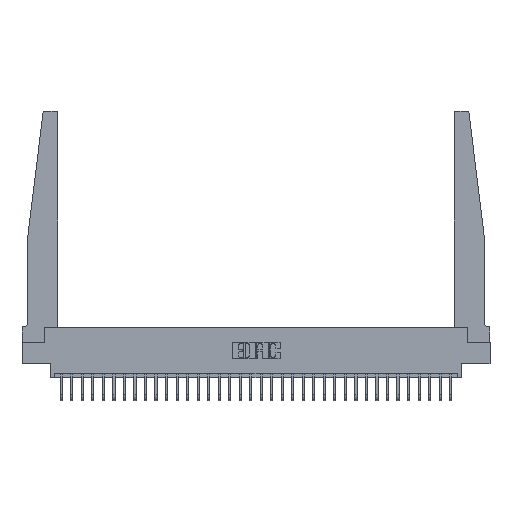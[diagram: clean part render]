
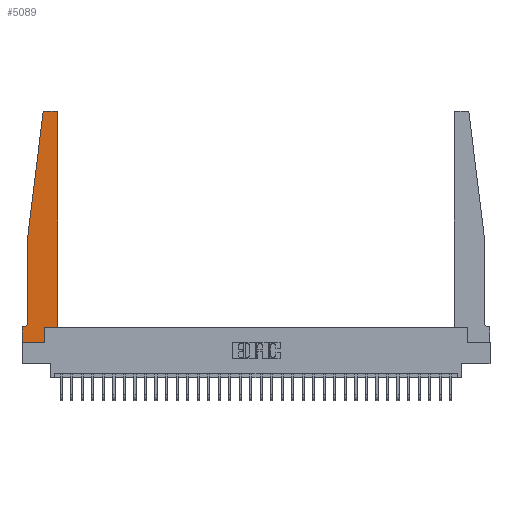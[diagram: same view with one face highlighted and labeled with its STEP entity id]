
A CAD part, top view. The second image highlights one B-rep face of the part: STEP entity #5089.
In plain terms, the highlighted planar face has unit normal (0, 0, 1).
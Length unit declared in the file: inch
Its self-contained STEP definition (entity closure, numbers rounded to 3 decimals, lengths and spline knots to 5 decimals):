
#339 = EDGE_CURVE ( 'NONE', #12382, #13331, #5246, .T. ) ;
#435 = FACE_OUTER_BOUND ( 'NONE', #11037, .T. ) ;
#787 = VERTEX_POINT ( 'NONE', #13876 ) ;
#1218 = VECTOR ( 'NONE', #23443, 39.37008 ) ;
#1477 = CARTESIAN_POINT ( 'NONE',  ( 0.395, 2.72, 0.37 ) ) ;
#1482 = DIRECTION ( 'NONE',  ( -1., 0., 0. ) ) ;
#1632 = CARTESIAN_POINT ( 'NONE',  ( 0., 0., 0.37 ) ) ;
#1955 = LINE ( 'NONE', #21192, #1218 ) ;
#2111 = ORIENTED_EDGE ( 'NONE', *, *, #27440, .T. ) ;
#2190 = LINE ( 'NONE', #15433, #6166 ) ;
#2281 = EDGE_CURVE ( 'NONE', #15164, #2390, #3346, .T. ) ;
#2390 = VERTEX_POINT ( 'NONE', #8690 ) ;
#2768 = CARTESIAN_POINT ( 'NONE',  ( 0.425, 2.72, 0.37 ) ) ;
#2798 = VERTEX_POINT ( 'NONE', #14584 ) ;
#3346 = LINE ( 'NONE', #19390, #26452 ) ;
#3579 = CARTESIAN_POINT ( 'NONE',  ( 0.2605, 0.18, 0.37 ) ) ;
#3644 = EDGE_CURVE ( 'NONE', #13331, #2798, #2190, .T. ) ;
#3822 = DIRECTION ( 'NONE',  ( 1., 0., 0. ) ) ;
#3839 = VECTOR ( 'NONE', #19632, 39.37008 ) ;
#3952 = DIRECTION ( 'NONE',  ( 0., 0., -1. ) ) ;
#4383 = ORIENTED_EDGE ( 'NONE', *, *, #16324, .T. ) ;
#4418 = DIRECTION ( 'NONE',  ( 0., 0., 1. ) ) ;
#4442 = ORIENTED_EDGE ( 'NONE', *, *, #9662, .T. ) ;
#4930 = CARTESIAN_POINT ( 'NONE',  ( 0.065, 1.25, 0.37 ) ) ;
#5016 = VERTEX_POINT ( 'NONE', #24161 ) ;
#5089 = ADVANCED_FACE ( 'NONE', ( #435 ), #15569, .T. ) ;
#5246 = LINE ( 'NONE', #3579, #22359 ) ;
#5272 = AXIS2_PLACEMENT_3D ( 'NONE', #22437, #9103, #24684 ) ;
#5592 = ORIENTED_EDGE ( 'NONE', *, *, #10603, .T. ) ;
#6166 = VECTOR ( 'NONE', #11150, 39.37008 ) ;
#7247 = CARTESIAN_POINT ( 'NONE',  ( 0.395, 2.75, 0.37 ) ) ;
#7549 = ORIENTED_EDGE ( 'NONE', *, *, #24615, .T. ) ;
#8267 = CARTESIAN_POINT ( 'NONE',  ( 0.065, 1.25, 0.37 ) ) ;
#8557 = LINE ( 'NONE', #25179, #19693 ) ;
#8690 = CARTESIAN_POINT ( 'NONE',  ( 0., 0.1875, 0.37 ) ) ;
#9103 = DIRECTION ( 'NONE',  ( 0., 0., 1. ) ) ;
#9288 = CARTESIAN_POINT ( 'NONE',  ( 0.25, 2.75, 0.37 ) ) ;
#9388 = CARTESIAN_POINT ( 'NONE',  ( 0.2605, 0., 0.37 ) ) ;
#9662 = EDGE_CURVE ( 'NONE', #21662, #10698, #18892, .T. ) ;
#10601 = CIRCLE ( 'NONE', #15765, 0.05 ) ;
#10603 = EDGE_CURVE ( 'NONE', #5016, #787, #27200, .T. ) ;
#10657 = EDGE_CURVE ( 'NONE', #10698, #5016, #14660, .T. ) ;
#10698 = VERTEX_POINT ( 'NONE', #7247 ) ;
#11037 = EDGE_LOOP ( 'NONE', ( #26169, #5592, #16190, #2111, #7549, #25469, #4383, #26163, #25231, #12651, #22467, #4442 ) ) ;
#11150 = DIRECTION ( 'NONE',  ( 1., 0., 0. ) ) ;
#11253 = LINE ( 'NONE', #4930, #21707 ) ;
#12382 = VERTEX_POINT ( 'NONE', #9388 ) ;
#12464 = CARTESIAN_POINT ( 'NONE',  ( 0.065, 0.2375, 0.37 ) ) ;
#12651 = ORIENTED_EDGE ( 'NONE', *, *, #3644, .T. ) ;
#12774 = LINE ( 'NONE', #13420, #18703 ) ;
#13331 = VERTEX_POINT ( 'NONE', #28019 ) ;
#13420 = CARTESIAN_POINT ( 'NONE',  ( 0., 0., 0.37 ) ) ;
#13876 = CARTESIAN_POINT ( 'NONE',  ( 0.24675, 2.72367, 0.37 ) ) ;
#14417 = AXIS2_PLACEMENT_3D ( 'NONE', #1477, #17260, #3822 ) ;
#14584 = CARTESIAN_POINT ( 'NONE',  ( 0.425, 0.18, 0.37 ) ) ;
#14660 = LINE ( 'NONE', #9288, #25820 ) ;
#15164 = VERTEX_POINT ( 'NONE', #19378 ) ;
#15433 = CARTESIAN_POINT ( 'NONE',  ( 0.425, 0.18, 0.37 ) ) ;
#15569 = PLANE ( 'NONE',  #17162 ) ;
#15765 = AXIS2_PLACEMENT_3D ( 'NONE', #17368, #3952, #19611 ) ;
#15772 = LINE ( 'NONE', #1632, #3839 ) ;
#15847 = VERTEX_POINT ( 'NONE', #18084 ) ;
#16190 = ORIENTED_EDGE ( 'NONE', *, *, #25506, .T. ) ;
#16324 = EDGE_CURVE ( 'NONE', #2390, #15847, #15772, .T. ) ;
#17162 = AXIS2_PLACEMENT_3D ( 'NONE', #24457, #4418, #20051 ) ;
#17260 = DIRECTION ( 'NONE',  ( 0., 0., 1. ) ) ;
#17368 = CARTESIAN_POINT ( 'NONE',  ( 0.015, 0.2375, 0.37 ) ) ;
#18084 = CARTESIAN_POINT ( 'NONE',  ( 0., 0., 0.37 ) ) ;
#18703 = VECTOR ( 'NONE', #28998, 39.37008 ) ;
#18892 = CIRCLE ( 'NONE', #14417, 0.03 ) ;
#19264 = DIRECTION ( 'NONE',  ( 0., 1., 0. ) ) ;
#19378 = CARTESIAN_POINT ( 'NONE',  ( 0.015, 0.1875, 0.37 ) ) ;
#19390 = CARTESIAN_POINT ( 'NONE',  ( 0.065, 0.1875, 0.37 ) ) ;
#19611 = DIRECTION ( 'NONE',  ( -1., 0., 0. ) ) ;
#19632 = DIRECTION ( 'NONE',  ( 0., -1., 0. ) ) ;
#19693 = VECTOR ( 'NONE', #27398, 39.37008 ) ;
#20051 = DIRECTION ( 'NONE',  ( 1., 0., 0. ) ) ;
#20358 = VERTEX_POINT ( 'NONE', #12464 ) ;
#21192 = CARTESIAN_POINT ( 'NONE',  ( 0.065, 1.25, 0.37 ) ) ;
#21662 = VERTEX_POINT ( 'NONE', #2768 ) ;
#21707 = VECTOR ( 'NONE', #25409, 39.37008 ) ;
#22359 = VECTOR ( 'NONE', #19264, 39.37008 ) ;
#22437 = CARTESIAN_POINT ( 'NONE',  ( 0.27653, 2.72, 0.37 ) ) ;
#22467 = ORIENTED_EDGE ( 'NONE', *, *, #24278, .T. ) ;
#23201 = EDGE_CURVE ( 'NONE', #15847, #12382, #12774, .T. ) ;
#23443 = DIRECTION ( 'NONE',  ( 0., -1., 0. ) ) ;
#23915 = VERTEX_POINT ( 'NONE', #8267 ) ;
#24161 = CARTESIAN_POINT ( 'NONE',  ( 0.27653, 2.75, 0.37 ) ) ;
#24278 = EDGE_CURVE ( 'NONE', #2798, #21662, #8557, .T. ) ;
#24457 = CARTESIAN_POINT ( 'NONE',  ( 0., 0.1875, 0.37 ) ) ;
#24615 = EDGE_CURVE ( 'NONE', #20358, #15164, #10601, .T. ) ;
#24684 = DIRECTION ( 'NONE',  ( 1., 0., 0. ) ) ;
#24869 = DIRECTION ( 'NONE',  ( -1., 0., 0. ) ) ;
#25179 = CARTESIAN_POINT ( 'NONE',  ( 0.425, 0.18, 0.37 ) ) ;
#25231 = ORIENTED_EDGE ( 'NONE', *, *, #339, .T. ) ;
#25409 = DIRECTION ( 'NONE',  ( -0.122, -0.992, 0. ) ) ;
#25469 = ORIENTED_EDGE ( 'NONE', *, *, #2281, .T. ) ;
#25506 = EDGE_CURVE ( 'NONE', #787, #23915, #11253, .T. ) ;
#25820 = VECTOR ( 'NONE', #24869, 39.37008 ) ;
#26163 = ORIENTED_EDGE ( 'NONE', *, *, #23201, .T. ) ;
#26169 = ORIENTED_EDGE ( 'NONE', *, *, #10657, .T. ) ;
#26452 = VECTOR ( 'NONE', #1482, 39.37008 ) ;
#27200 = CIRCLE ( 'NONE', #5272, 0.03 ) ;
#27398 = DIRECTION ( 'NONE',  ( 0., 1., 0. ) ) ;
#27440 = EDGE_CURVE ( 'NONE', #23915, #20358, #1955, .T. ) ;
#28019 = CARTESIAN_POINT ( 'NONE',  ( 0.2605, 0.18, 0.37 ) ) ;
#28998 = DIRECTION ( 'NONE',  ( 1., 0., 0. ) ) ;
